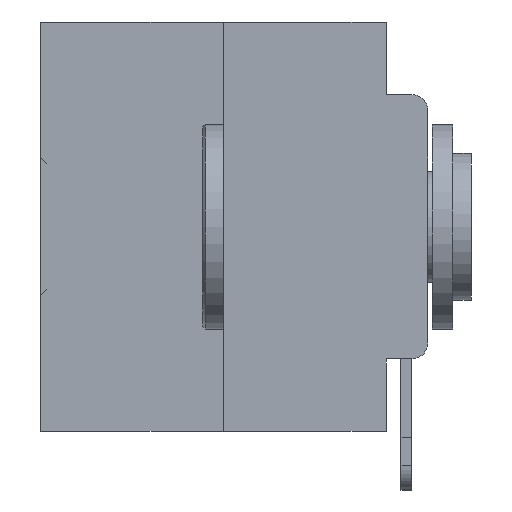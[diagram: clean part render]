
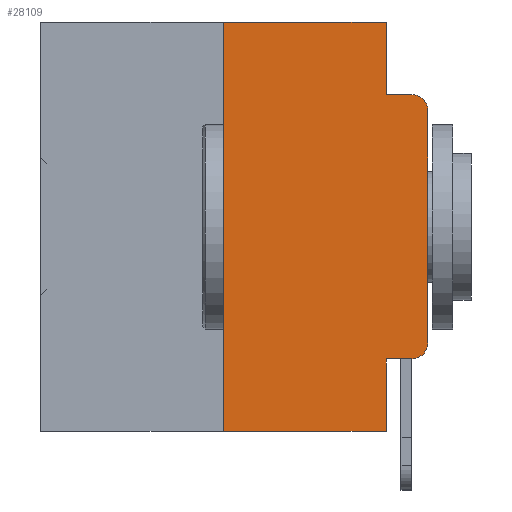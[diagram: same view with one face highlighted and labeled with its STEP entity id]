
A CAD part, left-side view. The second image highlights one B-rep face of the part: STEP entity #28109.
In plain terms, the highlighted planar face has unit normal (-1, 0, 0).
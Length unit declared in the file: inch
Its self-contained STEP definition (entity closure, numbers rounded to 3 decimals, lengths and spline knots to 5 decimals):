
#330 = ORIENTED_EDGE ( 'NONE', *, *, #24697, .T. ) ;
#1772 = ORIENTED_EDGE ( 'NONE', *, *, #7742, .T. ) ;
#2505 = DIRECTION ( 'NONE',  ( -1., 0., 0. ) ) ;
#2701 = DIRECTION ( 'NONE',  ( 0., 0., -1. ) ) ;
#3787 = CARTESIAN_POINT ( 'NONE',  ( 0., 0.473, 0. ) ) ;
#4051 = VECTOR ( 'NONE', #9339, 39.37008 ) ;
#4739 = ORIENTED_EDGE ( 'NONE', *, *, #13262, .T. ) ;
#5615 = VERTEX_POINT ( 'NONE', #10588 ) ;
#5839 = LINE ( 'NONE', #26930, #33414 ) ;
#5939 = VECTOR ( 'NONE', #34022, 39.37008 ) ;
#6133 = CARTESIAN_POINT ( 'NONE',  ( 0., 0., -0.1085 ) ) ;
#6775 = VERTEX_POINT ( 'NONE', #32919 ) ;
#6943 = CARTESIAN_POINT ( 'NONE',  ( 0., 0.02, -0.1085 ) ) ;
#7295 = CARTESIAN_POINT ( 'NONE',  ( 0., 0., 0. ) ) ;
#7742 = EDGE_CURVE ( 'NONE', #23968, #6775, #12239, .T. ) ;
#7854 = CARTESIAN_POINT ( 'NONE',  ( 0., 0., -0.3915 ) ) ;
#9339 = DIRECTION ( 'NONE',  ( 0., -1., 0. ) ) ;
#9714 = DIRECTION ( 'NONE',  ( 0., 0., -1. ) ) ;
#10116 = FACE_OUTER_BOUND ( 'NONE', #14423, .T. ) ;
#10506 = VECTOR ( 'NONE', #15606, 39.37008 ) ;
#10533 = CARTESIAN_POINT ( 'NONE',  ( 0., 0.25, 0. ) ) ;
#10588 = CARTESIAN_POINT ( 'NONE',  ( 0., 0.25, 0. ) ) ;
#11600 = LINE ( 'NONE', #10533, #12481 ) ;
#12239 = LINE ( 'NONE', #20308, #4051 ) ;
#12481 = VECTOR ( 'NONE', #21759, 39.37008 ) ;
#12920 = CARTESIAN_POINT ( 'NONE',  ( 0., 0.25, -0.5 ) ) ;
#13262 = EDGE_CURVE ( 'NONE', #30225, #22064, #34414, .T. ) ;
#13473 = ORIENTED_EDGE ( 'NONE', *, *, #19365, .F. ) ;
#13743 = DIRECTION ( 'NONE',  ( 0., 0., -1. ) ) ;
#14165 = VECTOR ( 'NONE', #31886, 39.37008 ) ;
#14423 = EDGE_LOOP ( 'NONE', ( #18919, #330, #29537, #16200, #13473, #25613, #1772, #16214, #4739, #27437 ) ) ;
#15383 = CARTESIAN_POINT ( 'NONE',  ( 0., 0.051, -0.4115 ) ) ;
#15606 = DIRECTION ( 'NONE',  ( 0., 0., 1. ) ) ;
#16200 = ORIENTED_EDGE ( 'NONE', *, *, #24119, .F. ) ;
#16214 = ORIENTED_EDGE ( 'NONE', *, *, #20719, .F. ) ;
#16439 = PLANE ( 'NONE',  #27886 ) ;
#16627 = EDGE_CURVE ( 'NONE', #21406, #25756, #25173, .T. ) ;
#17177 = VERTEX_POINT ( 'NONE', #17995 ) ;
#17995 = CARTESIAN_POINT ( 'NONE',  ( 0., 0.051, -0.0885 ) ) ;
#18521 = EDGE_CURVE ( 'NONE', #23968, #5615, #11600, .T. ) ;
#18741 = VECTOR ( 'NONE', #30857, 39.37008 ) ;
#18919 = ORIENTED_EDGE ( 'NONE', *, *, #16627, .T. ) ;
#19008 = CARTESIAN_POINT ( 'NONE',  ( 0., 0.02, -0.3915 ) ) ;
#19207 = DIRECTION ( 'NONE',  ( 1., 0., 0. ) ) ;
#19365 = EDGE_CURVE ( 'NONE', #5615, #20520, #29622, .T. ) ;
#19915 = CARTESIAN_POINT ( 'NONE',  ( 0., 0.051, -0.0885 ) ) ;
#20308 = CARTESIAN_POINT ( 'NONE',  ( 0., 0.473, -0.5 ) ) ;
#20393 = AXIS2_PLACEMENT_3D ( 'NONE', #19008, #2505, #21782 ) ;
#20520 = VERTEX_POINT ( 'NONE', #20594 ) ;
#20594 = CARTESIAN_POINT ( 'NONE',  ( 0., 0.051, 0. ) ) ;
#20719 = EDGE_CURVE ( 'NONE', #30225, #6775, #5839, .T. ) ;
#20768 = EDGE_CURVE ( 'NONE', #22064, #21406, #25229, .T. ) ;
#21406 = VERTEX_POINT ( 'NONE', #7854 ) ;
#21759 = DIRECTION ( 'NONE',  ( 0., 0., 1. ) ) ;
#21782 = DIRECTION ( 'NONE',  ( 0., 0., -1. ) ) ;
#22064 = VERTEX_POINT ( 'NONE', #26167 ) ;
#22930 = CARTESIAN_POINT ( 'NONE',  ( 0., 0.051, -0.4115 ) ) ;
#23968 = VERTEX_POINT ( 'NONE', #12920 ) ;
#24119 = EDGE_CURVE ( 'NONE', #20520, #17177, #33274, .T. ) ;
#24697 = EDGE_CURVE ( 'NONE', #25756, #30169, #28020, .T. ) ;
#25173 = LINE ( 'NONE', #7295, #10506 ) ;
#25229 = CIRCLE ( 'NONE', #20393, 0.02 ) ;
#25613 = ORIENTED_EDGE ( 'NONE', *, *, #18521, .F. ) ;
#25756 = VERTEX_POINT ( 'NONE', #6133 ) ;
#25936 = VECTOR ( 'NONE', #13743, 39.37008 ) ;
#26167 = CARTESIAN_POINT ( 'NONE',  ( 0., 0.02, -0.4115 ) ) ;
#26206 = DIRECTION ( 'NONE',  ( -1., 0., 0. ) ) ;
#26930 = CARTESIAN_POINT ( 'NONE',  ( 0., 0.051, 0. ) ) ;
#27437 = ORIENTED_EDGE ( 'NONE', *, *, #20768, .T. ) ;
#27886 = AXIS2_PLACEMENT_3D ( 'NONE', #35002, #19207, #2701 ) ;
#28020 = CIRCLE ( 'NONE', #32473, 0.02 ) ;
#28109 = ADVANCED_FACE ( 'NONE', ( #10116 ), #16439, .F. ) ;
#28284 = EDGE_CURVE ( 'NONE', #17177, #30169, #33373, .T. ) ;
#29537 = ORIENTED_EDGE ( 'NONE', *, *, #28284, .F. ) ;
#29622 = LINE ( 'NONE', #3787, #5939 ) ;
#30169 = VERTEX_POINT ( 'NONE', #33627 ) ;
#30225 = VERTEX_POINT ( 'NONE', #22930 ) ;
#30241 = CARTESIAN_POINT ( 'NONE',  ( 0., 0.051, 0. ) ) ;
#30857 = DIRECTION ( 'NONE',  ( 0., -1., 0. ) ) ;
#31886 = DIRECTION ( 'NONE',  ( 0., -1., 0. ) ) ;
#32473 = AXIS2_PLACEMENT_3D ( 'NONE', #6943, #26206, #9714 ) ;
#32919 = CARTESIAN_POINT ( 'NONE',  ( 0., 0.051, -0.5 ) ) ;
#33274 = LINE ( 'NONE', #30241, #25936 ) ;
#33373 = LINE ( 'NONE', #19915, #18741 ) ;
#33414 = VECTOR ( 'NONE', #35232, 39.37008 ) ;
#33627 = CARTESIAN_POINT ( 'NONE',  ( 0., 0.02, -0.0885 ) ) ;
#34022 = DIRECTION ( 'NONE',  ( 0., -1., 0. ) ) ;
#34414 = LINE ( 'NONE', #15383, #14165 ) ;
#35002 = CARTESIAN_POINT ( 'NONE',  ( 0., 0.473, 0. ) ) ;
#35232 = DIRECTION ( 'NONE',  ( 0., 0., -1. ) ) ;
